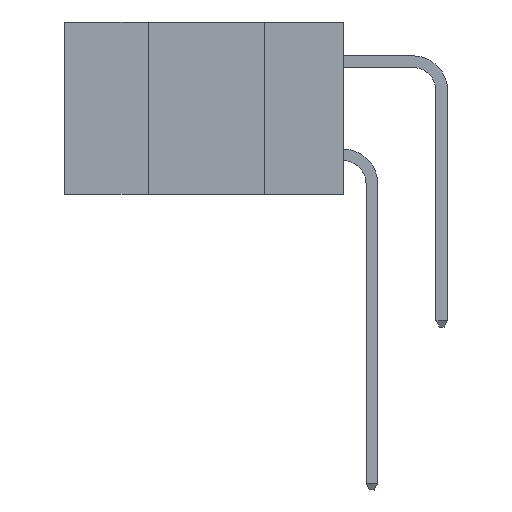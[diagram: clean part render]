
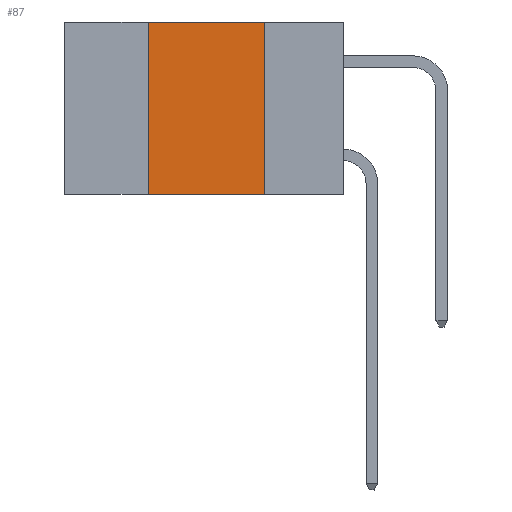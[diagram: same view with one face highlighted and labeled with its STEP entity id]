
A CAD part, left-side view. The second image highlights one B-rep face of the part: STEP entity #87.
In plain terms, the highlighted planar face has unit normal (-1, 0, 0).
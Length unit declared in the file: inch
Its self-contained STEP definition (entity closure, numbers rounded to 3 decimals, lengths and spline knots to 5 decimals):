
#2 = VECTOR ( 'NONE', #16687, 39.37008 ) ;
#87 = ADVANCED_FACE ( 'NONE', ( #6623 ), #6869, .F. ) ;
#347 = VERTEX_POINT ( 'NONE', #3200 ) ;
#919 = AXIS2_PLACEMENT_3D ( 'NONE', #15053, #18001, #8016 ) ;
#2074 = EDGE_LOOP ( 'NONE', ( #4039, #5896, #7232, #2837 ) ) ;
#2127 = CARTESIAN_POINT ( 'NONE',  ( 0., 0.6, 0. ) ) ;
#2837 = ORIENTED_EDGE ( 'NONE', *, *, #5803, .T. ) ;
#3200 = CARTESIAN_POINT ( 'NONE',  ( 0., 0.17, -0.37 ) ) ;
#4039 = ORIENTED_EDGE ( 'NONE', *, *, #13886, .F. ) ;
#4415 = LINE ( 'NONE', #6844, #2 ) ;
#4593 = DIRECTION ( 'NONE',  ( 0., -1., 0. ) ) ;
#4808 = VECTOR ( 'NONE', #10433, 39.37008 ) ;
#5419 = CARTESIAN_POINT ( 'NONE',  ( 0., 0.17, 0. ) ) ;
#5610 = CARTESIAN_POINT ( 'NONE',  ( 0., 0.42, -0.37 ) ) ;
#5803 = EDGE_CURVE ( 'NONE', #14450, #347, #9155, .T. ) ;
#5896 = ORIENTED_EDGE ( 'NONE', *, *, #15294, .F. ) ;
#6248 = CARTESIAN_POINT ( 'NONE',  ( 0., 0.42, 0. ) ) ;
#6623 = FACE_OUTER_BOUND ( 'NONE', #2074, .T. ) ;
#6844 = CARTESIAN_POINT ( 'NONE',  ( 0., 0.42, 0. ) ) ;
#6869 = PLANE ( 'NONE',  #919 ) ;
#6939 = VECTOR ( 'NONE', #4593, 39.37008 ) ;
#7232 = ORIENTED_EDGE ( 'NONE', *, *, #13696, .F. ) ;
#8016 = DIRECTION ( 'NONE',  ( 0., 0., -1. ) ) ;
#8555 = LINE ( 'NONE', #2127, #4808 ) ;
#8807 = VECTOR ( 'NONE', #14393, 39.37008 ) ;
#8818 = CARTESIAN_POINT ( 'NONE',  ( 0., 0.6, -0.37 ) ) ;
#9155 = LINE ( 'NONE', #8818, #6939 ) ;
#10343 = LINE ( 'NONE', #15789, #8807 ) ;
#10433 = DIRECTION ( 'NONE',  ( 0., -1., 0. ) ) ;
#11268 = VERTEX_POINT ( 'NONE', #6248 ) ;
#12835 = VERTEX_POINT ( 'NONE', #5419 ) ;
#13696 = EDGE_CURVE ( 'NONE', #14450, #11268, #4415, .T. ) ;
#13886 = EDGE_CURVE ( 'NONE', #12835, #347, #10343, .T. ) ;
#14393 = DIRECTION ( 'NONE',  ( 0., 0., -1. ) ) ;
#14450 = VERTEX_POINT ( 'NONE', #5610 ) ;
#15053 = CARTESIAN_POINT ( 'NONE',  ( 0., 0.6, 0. ) ) ;
#15294 = EDGE_CURVE ( 'NONE', #11268, #12835, #8555, .T. ) ;
#15789 = CARTESIAN_POINT ( 'NONE',  ( 0., 0.17, 0. ) ) ;
#16687 = DIRECTION ( 'NONE',  ( 0., 0., 1. ) ) ;
#18001 = DIRECTION ( 'NONE',  ( 1., 0., 0. ) ) ;
